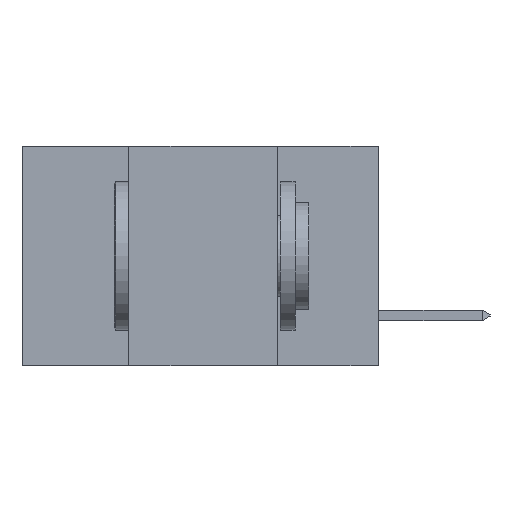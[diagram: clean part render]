
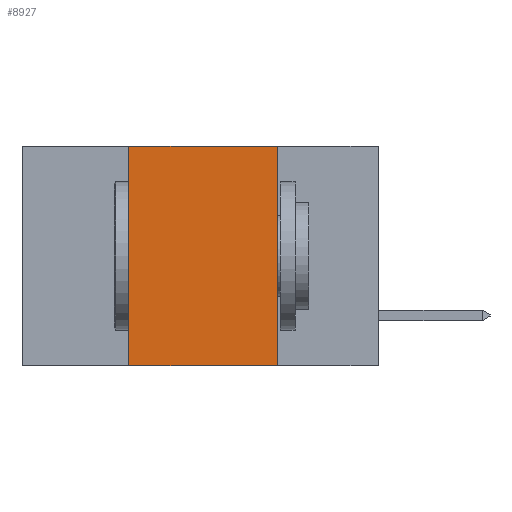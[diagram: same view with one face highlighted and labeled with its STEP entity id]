
A CAD part, left-side view. The second image highlights one B-rep face of the part: STEP entity #8927.
In plain terms, the highlighted planar face has unit normal (-1, 0, 0).
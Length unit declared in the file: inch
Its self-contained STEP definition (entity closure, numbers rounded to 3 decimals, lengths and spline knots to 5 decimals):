
#962 = CARTESIAN_POINT ( 'NONE',  ( 0., 0.42, -0.37 ) ) ;
#1191 = VERTEX_POINT ( 'NONE', #6570 ) ;
#1290 = PLANE ( 'NONE',  #7674 ) ;
#1486 = EDGE_CURVE ( 'NONE', #1191, #7232, #3808, .T. ) ;
#1870 = ORIENTED_EDGE ( 'NONE', *, *, #1486, .F. ) ;
#2848 = DIRECTION ( 'NONE',  ( 1., 0., 0. ) ) ;
#3072 = VECTOR ( 'NONE', #9536, 39.37008 ) ;
#3154 = CARTESIAN_POINT ( 'NONE',  ( 0., 0.6, 0. ) ) ;
#3170 = CARTESIAN_POINT ( 'NONE',  ( 0., 0.17, -0.37 ) ) ;
#3190 = DIRECTION ( 'NONE',  ( 0., -1., 0. ) ) ;
#3491 = EDGE_CURVE ( 'NONE', #7105, #1191, #6846, .T. ) ;
#3576 = VECTOR ( 'NONE', #9346, 39.37008 ) ;
#3808 = LINE ( 'NONE', #6389, #3576 ) ;
#4486 = EDGE_CURVE ( 'NONE', #9230, #7105, #9628, .T. ) ;
#4657 = VECTOR ( 'NONE', #3190, 39.37008 ) ;
#5774 = CARTESIAN_POINT ( 'NONE',  ( 0., 0.42, -0.37 ) ) ;
#5806 = CARTESIAN_POINT ( 'NONE',  ( 0., 0.6, -0.37 ) ) ;
#5973 = CARTESIAN_POINT ( 'NONE',  ( 0., 0.42, 0. ) ) ;
#6048 = DIRECTION ( 'NONE',  ( 0., 0., 1. ) ) ;
#6389 = CARTESIAN_POINT ( 'NONE',  ( 0., 0.17, -0.37 ) ) ;
#6418 = ORIENTED_EDGE ( 'NONE', *, *, #4486, .F. ) ;
#6553 = EDGE_LOOP ( 'NONE', ( #1870, #8077, #6418, #8758 ) ) ;
#6570 = CARTESIAN_POINT ( 'NONE',  ( 0., 0.17, 0. ) ) ;
#6846 = LINE ( 'NONE', #3154, #4657 ) ;
#6957 = EDGE_CURVE ( 'NONE', #9230, #7232, #7015, .T. ) ;
#7015 = LINE ( 'NONE', #5806, #3072 ) ;
#7105 = VERTEX_POINT ( 'NONE', #5973 ) ;
#7232 = VERTEX_POINT ( 'NONE', #3170 ) ;
#7307 = CARTESIAN_POINT ( 'NONE',  ( 0., 0.6, 0. ) ) ;
#7674 = AXIS2_PLACEMENT_3D ( 'NONE', #7307, #2848, #8059 ) ;
#7885 = VECTOR ( 'NONE', #6048, 39.37008 ) ;
#8059 = DIRECTION ( 'NONE',  ( 0., 0., -1. ) ) ;
#8077 = ORIENTED_EDGE ( 'NONE', *, *, #3491, .F. ) ;
#8758 = ORIENTED_EDGE ( 'NONE', *, *, #6957, .T. ) ;
#8927 = ADVANCED_FACE ( 'NONE', ( #9531 ), #1290, .F. ) ;
#9230 = VERTEX_POINT ( 'NONE', #962 ) ;
#9346 = DIRECTION ( 'NONE',  ( 0., 0., -1. ) ) ;
#9531 = FACE_OUTER_BOUND ( 'NONE', #6553, .T. ) ;
#9536 = DIRECTION ( 'NONE',  ( 0., -1., 0. ) ) ;
#9628 = LINE ( 'NONE', #5774, #7885 ) ;
